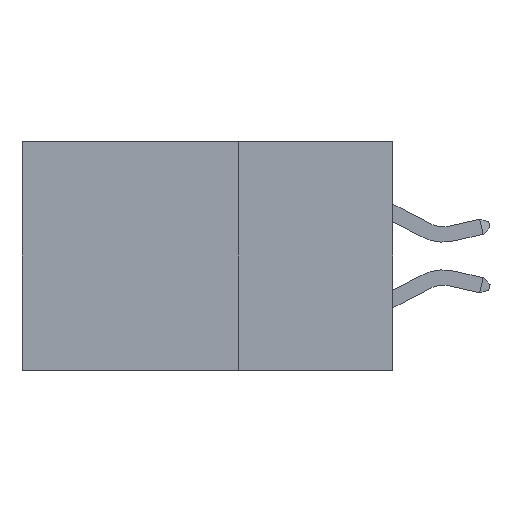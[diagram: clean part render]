
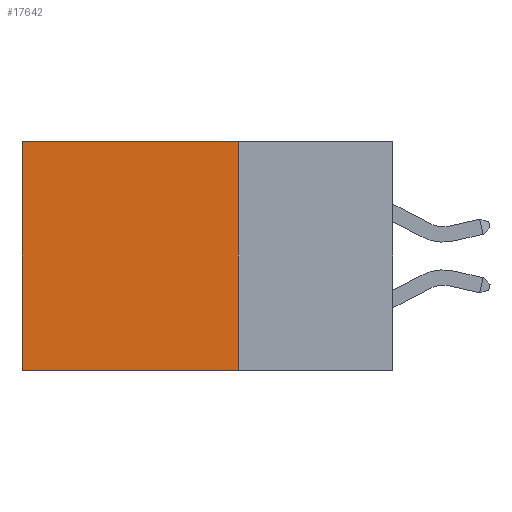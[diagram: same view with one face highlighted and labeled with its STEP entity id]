
A CAD part, left-side view. The second image highlights one B-rep face of the part: STEP entity #17642.
In plain terms, the highlighted planar face has unit normal (-1, 0, 0).
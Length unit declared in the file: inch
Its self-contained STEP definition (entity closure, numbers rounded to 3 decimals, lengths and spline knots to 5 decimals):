
#239 = CARTESIAN_POINT ( 'NONE',  ( 0.2875, 0.25, 0. ) ) ;
#912 = VERTEX_POINT ( 'NONE', #26745 ) ;
#1574 = FACE_OUTER_BOUND ( 'NONE', #29590, .T. ) ;
#5844 = ORIENTED_EDGE ( 'NONE', *, *, #38723, .T. ) ;
#6053 = EDGE_CURVE ( 'NONE', #16382, #28098, #12635, .T. ) ;
#6895 = ORIENTED_EDGE ( 'NONE', *, *, #6053, .T. ) ;
#10597 = VERTEX_POINT ( 'NONE', #40822 ) ;
#12635 = LINE ( 'NONE', #239, #26592 ) ;
#14428 = DIRECTION ( 'NONE',  ( 0., 0., -1. ) ) ;
#15256 = LINE ( 'NONE', #24220, #19379 ) ;
#16382 = VERTEX_POINT ( 'NONE', #37429 ) ;
#17642 = ADVANCED_FACE ( 'NONE', ( #1574 ), #40971, .F. ) ;
#19379 = VECTOR ( 'NONE', #14428, 39.37008 ) ;
#21181 = LINE ( 'NONE', #26848, #23732 ) ;
#23187 = CARTESIAN_POINT ( 'NONE',  ( 0.2875, 0.25, -0.37 ) ) ;
#23732 = VECTOR ( 'NONE', #26995, 39.37008 ) ;
#24220 = CARTESIAN_POINT ( 'NONE',  ( 0.2875, 0.6, 0. ) ) ;
#24448 = DIRECTION ( 'NONE',  ( 1., 0., 0. ) ) ;
#25349 = LINE ( 'NONE', #23187, #40377 ) ;
#26592 = VECTOR ( 'NONE', #39953, 39.37008 ) ;
#26745 = CARTESIAN_POINT ( 'NONE',  ( 0.2875, 0.25, -0.37 ) ) ;
#26848 = CARTESIAN_POINT ( 'NONE',  ( 0.2875, 0.25, 0. ) ) ;
#26995 = DIRECTION ( 'NONE',  ( 0., 0., -1. ) ) ;
#27354 = CARTESIAN_POINT ( 'NONE',  ( 0.2875, 0.6, 0. ) ) ;
#28098 = VERTEX_POINT ( 'NONE', #27354 ) ;
#29590 = EDGE_LOOP ( 'NONE', ( #5844, #41010, #29714, #6895 ) ) ;
#29714 = ORIENTED_EDGE ( 'NONE', *, *, #35141, .F. ) ;
#30847 = CARTESIAN_POINT ( 'NONE',  ( 0.2875, 0.25, 0. ) ) ;
#35141 = EDGE_CURVE ( 'NONE', #16382, #912, #21181, .T. ) ;
#35683 = EDGE_CURVE ( 'NONE', #912, #10597, #25349, .T. ) ;
#36853 = AXIS2_PLACEMENT_3D ( 'NONE', #30847, #24448, #37776 ) ;
#37429 = CARTESIAN_POINT ( 'NONE',  ( 0.2875, 0.25, 0. ) ) ;
#37776 = DIRECTION ( 'NONE',  ( 0., 0., -1. ) ) ;
#38723 = EDGE_CURVE ( 'NONE', #28098, #10597, #15256, .T. ) ;
#39953 = DIRECTION ( 'NONE',  ( 0., 1., 0. ) ) ;
#40377 = VECTOR ( 'NONE', #42901, 39.37008 ) ;
#40822 = CARTESIAN_POINT ( 'NONE',  ( 0.2875, 0.6, -0.37 ) ) ;
#40971 = PLANE ( 'NONE',  #36853 ) ;
#41010 = ORIENTED_EDGE ( 'NONE', *, *, #35683, .F. ) ;
#42901 = DIRECTION ( 'NONE',  ( 0., 1., 0. ) ) ;
